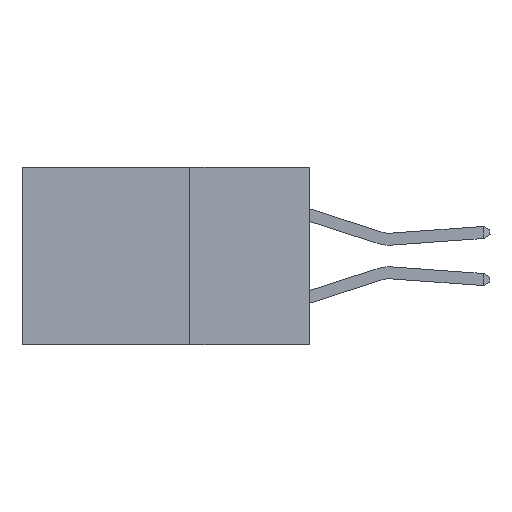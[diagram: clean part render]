
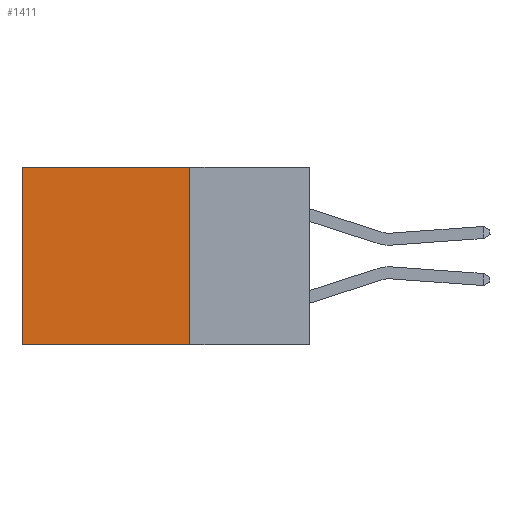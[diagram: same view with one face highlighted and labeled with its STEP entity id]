
A CAD part, left-side view. The second image highlights one B-rep face of the part: STEP entity #1411.
In plain terms, the highlighted planar face has unit normal (-1, 0, 0).
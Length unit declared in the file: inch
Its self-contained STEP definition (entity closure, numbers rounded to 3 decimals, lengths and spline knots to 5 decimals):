
#60 = DIRECTION ( 'NONE',  ( 0., 1., 0. ) ) ;
#131 = PLANE ( 'NONE',  #1171 ) ;
#394 = CARTESIAN_POINT ( 'NONE',  ( 0.298, 0.25, 0. ) ) ;
#528 = DIRECTION ( 'NONE',  ( 1., 0., 0. ) ) ;
#852 = CARTESIAN_POINT ( 'NONE',  ( 0.298, 0.25, -0.37 ) ) ;
#932 = VECTOR ( 'NONE', #1922, 39.37008 ) ;
#1171 = AXIS2_PLACEMENT_3D ( 'NONE', #2904, #528, #6934 ) ;
#1411 = ADVANCED_FACE ( 'NONE', ( #6532 ), #131, .F. ) ;
#1620 = CARTESIAN_POINT ( 'NONE',  ( 0.298, 0.6, 0. ) ) ;
#1658 = VECTOR ( 'NONE', #8702, 39.37008 ) ;
#1696 = VERTEX_POINT ( 'NONE', #2310 ) ;
#1922 = DIRECTION ( 'NONE',  ( 0., 1., 0. ) ) ;
#2310 = CARTESIAN_POINT ( 'NONE',  ( 0.298, 0.25, 0. ) ) ;
#2590 = CARTESIAN_POINT ( 'NONE',  ( 0.298, 0.25, 0. ) ) ;
#2794 = VECTOR ( 'NONE', #60, 39.37008 ) ;
#2904 = CARTESIAN_POINT ( 'NONE',  ( 0.298, 0.25, 0. ) ) ;
#2922 = EDGE_CURVE ( 'NONE', #1696, #3828, #7437, .T. ) ;
#3243 = EDGE_LOOP ( 'NONE', ( #7570, #9392, #4610, #5719 ) ) ;
#3828 = VERTEX_POINT ( 'NONE', #1620 ) ;
#3861 = LINE ( 'NONE', #394, #1658 ) ;
#3882 = VECTOR ( 'NONE', #10019, 39.37008 ) ;
#4093 = EDGE_CURVE ( 'NONE', #3828, #5591, #9660, .T. ) ;
#4610 = ORIENTED_EDGE ( 'NONE', *, *, #4976, .F. ) ;
#4666 = CARTESIAN_POINT ( 'NONE',  ( 0.298, 0.6, 0. ) ) ;
#4976 = EDGE_CURVE ( 'NONE', #1696, #10010, #3861, .T. ) ;
#5591 = VERTEX_POINT ( 'NONE', #6258 ) ;
#5719 = ORIENTED_EDGE ( 'NONE', *, *, #2922, .T. ) ;
#6258 = CARTESIAN_POINT ( 'NONE',  ( 0.298, 0.6, -0.37 ) ) ;
#6532 = FACE_OUTER_BOUND ( 'NONE', #3243, .T. ) ;
#6934 = DIRECTION ( 'NONE',  ( 0., 0., -1. ) ) ;
#7437 = LINE ( 'NONE', #2590, #932 ) ;
#7570 = ORIENTED_EDGE ( 'NONE', *, *, #4093, .T. ) ;
#8422 = CARTESIAN_POINT ( 'NONE',  ( 0.298, 0.25, -0.37 ) ) ;
#8702 = DIRECTION ( 'NONE',  ( 0., 0., -1. ) ) ;
#8919 = LINE ( 'NONE', #852, #2794 ) ;
#9392 = ORIENTED_EDGE ( 'NONE', *, *, #9594, .F. ) ;
#9594 = EDGE_CURVE ( 'NONE', #10010, #5591, #8919, .T. ) ;
#9660 = LINE ( 'NONE', #4666, #3882 ) ;
#10010 = VERTEX_POINT ( 'NONE', #8422 ) ;
#10019 = DIRECTION ( 'NONE',  ( 0., 0., -1. ) ) ;
